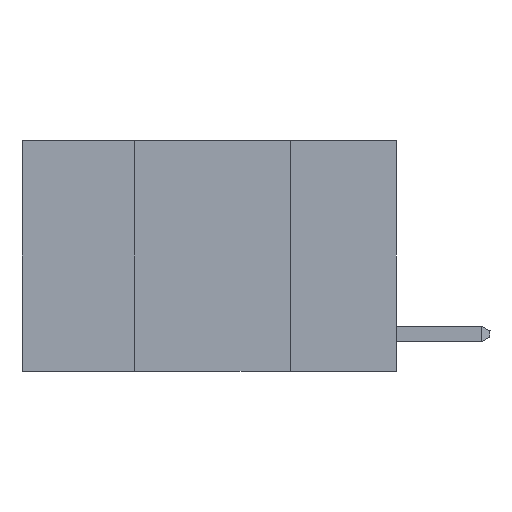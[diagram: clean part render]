
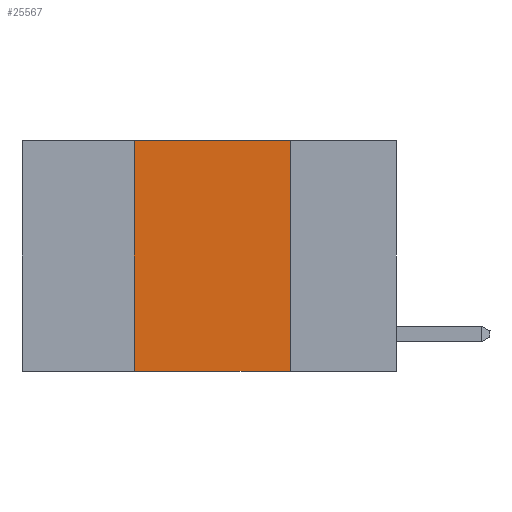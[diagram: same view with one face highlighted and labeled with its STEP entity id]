
A CAD part, left-side view. The second image highlights one B-rep face of the part: STEP entity #25567.
In plain terms, the highlighted planar face has unit normal (-1, 0, 0).
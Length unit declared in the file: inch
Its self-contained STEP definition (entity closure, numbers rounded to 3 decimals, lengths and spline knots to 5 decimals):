
#213 = CARTESIAN_POINT ( 'NONE',  ( 0., 0.6, 0. ) ) ;
#699 = VERTEX_POINT ( 'NONE', #2671 ) ;
#898 = LINE ( 'NONE', #26020, #7287 ) ;
#2671 = CARTESIAN_POINT ( 'NONE',  ( 0., 0.42, 0. ) ) ;
#3030 = DIRECTION ( 'NONE',  ( 0., -1., 0. ) ) ;
#3714 = CARTESIAN_POINT ( 'NONE',  ( 0., 0.17, 0. ) ) ;
#4288 = AXIS2_PLACEMENT_3D ( 'NONE', #8933, #27334, #11460 ) ;
#5692 = CARTESIAN_POINT ( 'NONE',  ( 0., 0.17, 0. ) ) ;
#6267 = EDGE_CURVE ( 'NONE', #699, #18774, #11547, .T. ) ;
#6924 = EDGE_CURVE ( 'NONE', #9999, #699, #898, .T. ) ;
#7255 = EDGE_LOOP ( 'NONE', ( #17306, #27146, #28019, #14206 ) ) ;
#7287 = VECTOR ( 'NONE', #19300, 39.37008 ) ;
#7911 = LINE ( 'NONE', #5692, #24509 ) ;
#8933 = CARTESIAN_POINT ( 'NONE',  ( 0., 0.6, 0. ) ) ;
#9999 = VERTEX_POINT ( 'NONE', #17299 ) ;
#10071 = EDGE_CURVE ( 'NONE', #9999, #27088, #21339, .T. ) ;
#11460 = DIRECTION ( 'NONE',  ( 0., 0., -1. ) ) ;
#11547 = LINE ( 'NONE', #213, #15822 ) ;
#14206 = ORIENTED_EDGE ( 'NONE', *, *, #10071, .T. ) ;
#14790 = DIRECTION ( 'NONE',  ( 0., 0., -1. ) ) ;
#15822 = VECTOR ( 'NONE', #3030, 39.37008 ) ;
#17000 = DIRECTION ( 'NONE',  ( 0., -1., 0. ) ) ;
#17299 = CARTESIAN_POINT ( 'NONE',  ( 0., 0.42, -0.37 ) ) ;
#17306 = ORIENTED_EDGE ( 'NONE', *, *, #21273, .F. ) ;
#18510 = PLANE ( 'NONE',  #4288 ) ;
#18774 = VERTEX_POINT ( 'NONE', #3714 ) ;
#19300 = DIRECTION ( 'NONE',  ( 0., 0., 1. ) ) ;
#20158 = FACE_OUTER_BOUND ( 'NONE', #7255, .T. ) ;
#21273 = EDGE_CURVE ( 'NONE', #18774, #27088, #7911, .T. ) ;
#21339 = LINE ( 'NONE', #28519, #27143 ) ;
#24290 = CARTESIAN_POINT ( 'NONE',  ( 0., 0.17, -0.37 ) ) ;
#24509 = VECTOR ( 'NONE', #14790, 39.37008 ) ;
#25567 = ADVANCED_FACE ( 'NONE', ( #20158 ), #18510, .F. ) ;
#26020 = CARTESIAN_POINT ( 'NONE',  ( 0., 0.42, 0. ) ) ;
#27088 = VERTEX_POINT ( 'NONE', #24290 ) ;
#27143 = VECTOR ( 'NONE', #17000, 39.37008 ) ;
#27146 = ORIENTED_EDGE ( 'NONE', *, *, #6267, .F. ) ;
#27334 = DIRECTION ( 'NONE',  ( 1., 0., 0. ) ) ;
#28019 = ORIENTED_EDGE ( 'NONE', *, *, #6924, .F. ) ;
#28519 = CARTESIAN_POINT ( 'NONE',  ( 0., 0.6, -0.37 ) ) ;
